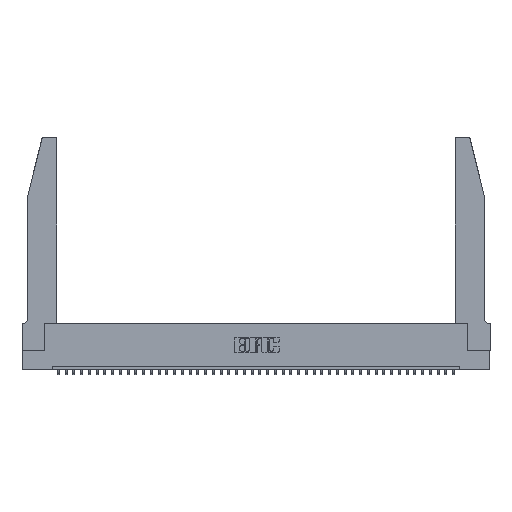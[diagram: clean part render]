
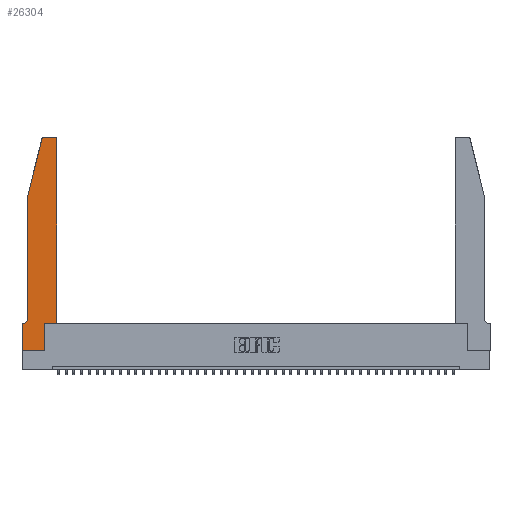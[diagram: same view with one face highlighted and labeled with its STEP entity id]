
A CAD part, top view. The second image highlights one B-rep face of the part: STEP entity #26304.
In plain terms, the highlighted planar face has unit normal (0, 0, 1).
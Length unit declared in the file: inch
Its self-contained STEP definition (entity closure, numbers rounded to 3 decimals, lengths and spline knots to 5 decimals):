
#226 = CARTESIAN_POINT ( 'NONE',  ( 0.4205, 2.75, 0.37 ) ) ;
#1016 = VERTEX_POINT ( 'NONE', #36404 ) ;
#1388 = ORIENTED_EDGE ( 'NONE', *, *, #26542, .T. ) ;
#2144 = EDGE_CURVE ( 'NONE', #1016, #8834, #4976, .T. ) ;
#2193 = DIRECTION ( 'NONE',  ( 0., 1., 0. ) ) ;
#2397 = EDGE_LOOP ( 'NONE', ( #36633, #14079, #4725, #24731, #15038, #29301, #1388, #26232, #14233, #16279, #41710, #15963 ) ) ;
#3685 = VECTOR ( 'NONE', #16309, 39.37008 ) ;
#3719 = CARTESIAN_POINT ( 'NONE',  ( 0., 0., 0.37 ) ) ;
#3724 = VECTOR ( 'NONE', #23255, 39.37008 ) ;
#4305 = EDGE_CURVE ( 'NONE', #21058, #9073, #31109, .T. ) ;
#4636 = VERTEX_POINT ( 'NONE', #16564 ) ;
#4725 = ORIENTED_EDGE ( 'NONE', *, *, #23732, .T. ) ;
#4976 = LINE ( 'NONE', #18378, #9552 ) ;
#5542 = CARTESIAN_POINT ( 'NONE',  ( 0.4505, 0.35, 0.37 ) ) ;
#5623 = VECTOR ( 'NONE', #16335, 39.37008 ) ;
#6907 = DIRECTION ( 'NONE',  ( 0., -1., 0. ) ) ;
#7123 = CARTESIAN_POINT ( 'NONE',  ( 0.25487, 2.72718, 0.37 ) ) ;
#8123 = DIRECTION ( 'NONE',  ( 1., 0., 0. ) ) ;
#8834 = VERTEX_POINT ( 'NONE', #27231 ) ;
#8971 = CARTESIAN_POINT ( 'NONE',  ( 0.0755, 0.42, 0.37 ) ) ;
#9073 = VERTEX_POINT ( 'NONE', #7123 ) ;
#9552 = VECTOR ( 'NONE', #2193, 39.37008 ) ;
#9720 = LINE ( 'NONE', #12401, #27710 ) ;
#10705 = EDGE_CURVE ( 'NONE', #4636, #1016, #9720, .T. ) ;
#11623 = EDGE_CURVE ( 'NONE', #19155, #21058, #13227, .T. ) ;
#11821 = PLANE ( 'NONE',  #41558 ) ;
#11954 = DIRECTION ( 'NONE',  ( 0., 0., 1. ) ) ;
#12049 = AXIS2_PLACEMENT_3D ( 'NONE', #29847, #16640, #39733 ) ;
#12401 = CARTESIAN_POINT ( 'NONE',  ( 0., 0., 0.37 ) ) ;
#12436 = LINE ( 'NONE', #29099, #17067 ) ;
#13227 = LINE ( 'NONE', #16199, #5623 ) ;
#13773 = AXIS2_PLACEMENT_3D ( 'NONE', #33488, #33200, #39895 ) ;
#13779 = VERTEX_POINT ( 'NONE', #13790 ) ;
#13790 = CARTESIAN_POINT ( 'NONE',  ( 0.0755, 2., 0.37 ) ) ;
#14079 = ORIENTED_EDGE ( 'NONE', *, *, #4305, .T. ) ;
#14233 = ORIENTED_EDGE ( 'NONE', *, *, #2144, .T. ) ;
#14752 = CARTESIAN_POINT ( 'NONE',  ( 0.4205, 2.72, 0.37 ) ) ;
#14991 = FACE_OUTER_BOUND ( 'NONE', #2397, .T. ) ;
#15038 = ORIENTED_EDGE ( 'NONE', *, *, #32232, .T. ) ;
#15455 = CARTESIAN_POINT ( 'NONE',  ( 0., 0.35, 0.37 ) ) ;
#15963 = ORIENTED_EDGE ( 'NONE', *, *, #26111, .T. ) ;
#16199 = CARTESIAN_POINT ( 'NONE',  ( 0.2605, 2.75, 0.37 ) ) ;
#16279 = ORIENTED_EDGE ( 'NONE', *, *, #19154, .T. ) ;
#16309 = DIRECTION ( 'NONE',  ( -1., 0., 0. ) ) ;
#16335 = DIRECTION ( 'NONE',  ( -1., 0., 0. ) ) ;
#16564 = CARTESIAN_POINT ( 'NONE',  ( 0., 0., 0.37 ) ) ;
#16589 = CARTESIAN_POINT ( 'NONE',  ( 0.0755, 0.35, 0.37 ) ) ;
#16640 = DIRECTION ( 'NONE',  ( 0., 0., -1. ) ) ;
#16936 = VERTEX_POINT ( 'NONE', #8971 ) ;
#16975 = LINE ( 'NONE', #16589, #3685 ) ;
#17063 = EDGE_CURVE ( 'NONE', #23781, #37770, #40426, .T. ) ;
#17067 = VECTOR ( 'NONE', #22958, 39.37008 ) ;
#18378 = CARTESIAN_POINT ( 'NONE',  ( 0.2865, 0.35, 0.37 ) ) ;
#18785 = DIRECTION ( 'NONE',  ( 1., 0., 0. ) ) ;
#19155 = VERTEX_POINT ( 'NONE', #226 ) ;
#19154 = EDGE_CURVE ( 'NONE', #8834, #23781, #12436, .T. ) ;
#20119 = CARTESIAN_POINT ( 'NONE',  ( 0.0755, 2., 0.37 ) ) ;
#20172 = CIRCLE ( 'NONE', #28208, 0.03 ) ;
#20806 = VECTOR ( 'NONE', #28877, 39.37008 ) ;
#21058 = VERTEX_POINT ( 'NONE', #40451 ) ;
#22958 = DIRECTION ( 'NONE',  ( 1., 0., 0. ) ) ;
#23255 = DIRECTION ( 'NONE',  ( 0., -1., 0. ) ) ;
#23732 = EDGE_CURVE ( 'NONE', #9073, #13779, #26613, .T. ) ;
#23781 = VERTEX_POINT ( 'NONE', #29453 ) ;
#24731 = ORIENTED_EDGE ( 'NONE', *, *, #29639, .T. ) ;
#26111 = EDGE_CURVE ( 'NONE', #37770, #19155, #20172, .T. ) ;
#26232 = ORIENTED_EDGE ( 'NONE', *, *, #10705, .T. ) ;
#26304 = ADVANCED_FACE ( 'NONE', ( #14991 ), #11821, .T. ) ;
#26542 = EDGE_CURVE ( 'NONE', #36686, #4636, #30919, .T. ) ;
#26613 = LINE ( 'NONE', #42282, #37871 ) ;
#27231 = CARTESIAN_POINT ( 'NONE',  ( 0.2865, 0.35, 0.37 ) ) ;
#27710 = VECTOR ( 'NONE', #41470, 39.37008 ) ;
#28155 = DIRECTION ( 'NONE',  ( 0., 0., 1. ) ) ;
#28157 = VERTEX_POINT ( 'NONE', #37676 ) ;
#28208 = AXIS2_PLACEMENT_3D ( 'NONE', #14752, #28155, #18785 ) ;
#28877 = DIRECTION ( 'NONE',  ( 0., 1., 0. ) ) ;
#29099 = CARTESIAN_POINT ( 'NONE',  ( 0.4505, 0.35, 0.37 ) ) ;
#29301 = ORIENTED_EDGE ( 'NONE', *, *, #31653, .T. ) ;
#29453 = CARTESIAN_POINT ( 'NONE',  ( 0.4505, 0.35, 0.37 ) ) ;
#29505 = VECTOR ( 'NONE', #6907, 39.37008 ) ;
#29639 = EDGE_CURVE ( 'NONE', #13779, #16936, #35168, .T. ) ;
#29847 = CARTESIAN_POINT ( 'NONE',  ( 0.0055, 0.42, 0.37 ) ) ;
#30919 = LINE ( 'NONE', #3719, #3724 ) ;
#31109 = CIRCLE ( 'NONE', #13773, 0.03 ) ;
#31240 = CARTESIAN_POINT ( 'NONE',  ( 0., 0.35, 0.37 ) ) ;
#31405 = CIRCLE ( 'NONE', #12049, 0.07 ) ;
#31653 = EDGE_CURVE ( 'NONE', #28157, #36686, #16975, .T. ) ;
#32232 = EDGE_CURVE ( 'NONE', #16936, #28157, #31405, .T. ) ;
#32400 = DIRECTION ( 'NONE',  ( -0.239, -0.971, 0. ) ) ;
#33200 = DIRECTION ( 'NONE',  ( 0., 0., 1. ) ) ;
#33488 = CARTESIAN_POINT ( 'NONE',  ( 0.284, 2.72, 0.37 ) ) ;
#35168 = LINE ( 'NONE', #20119, #29505 ) ;
#35213 = CARTESIAN_POINT ( 'NONE',  ( 0.4505, 2.72, 0.37 ) ) ;
#36404 = CARTESIAN_POINT ( 'NONE',  ( 0.2865, 0., 0.37 ) ) ;
#36633 = ORIENTED_EDGE ( 'NONE', *, *, #11623, .T. ) ;
#36686 = VERTEX_POINT ( 'NONE', #15455 ) ;
#37676 = CARTESIAN_POINT ( 'NONE',  ( 0.0055, 0.35, 0.37 ) ) ;
#37770 = VERTEX_POINT ( 'NONE', #35213 ) ;
#37871 = VECTOR ( 'NONE', #32400, 39.37008 ) ;
#39733 = DIRECTION ( 'NONE',  ( -1., 0., 0. ) ) ;
#39895 = DIRECTION ( 'NONE',  ( 1., 0., 0. ) ) ;
#40426 = LINE ( 'NONE', #5542, #20806 ) ;
#40451 = CARTESIAN_POINT ( 'NONE',  ( 0.284, 2.75, 0.37 ) ) ;
#41470 = DIRECTION ( 'NONE',  ( 1., 0., 0. ) ) ;
#41558 = AXIS2_PLACEMENT_3D ( 'NONE', #31240, #11954, #8123 ) ;
#41710 = ORIENTED_EDGE ( 'NONE', *, *, #17063, .T. ) ;
#42282 = CARTESIAN_POINT ( 'NONE',  ( 0.0755, 2., 0.37 ) ) ;
